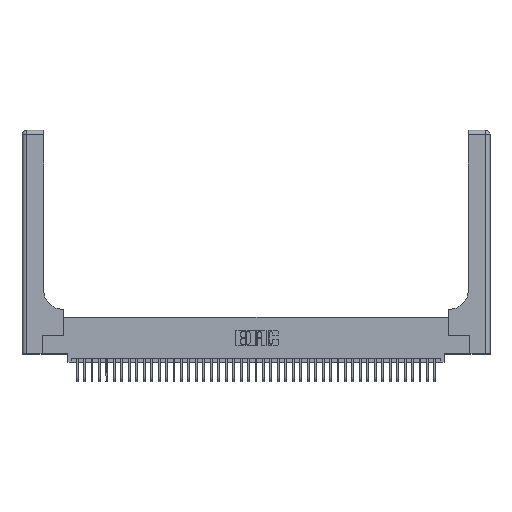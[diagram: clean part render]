
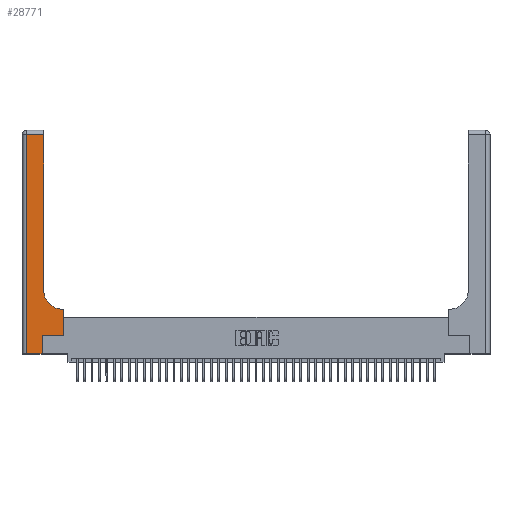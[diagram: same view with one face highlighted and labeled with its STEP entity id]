
A CAD part, top view. The second image highlights one B-rep face of the part: STEP entity #28771.
In plain terms, the highlighted planar face has unit normal (0, 0, 1).
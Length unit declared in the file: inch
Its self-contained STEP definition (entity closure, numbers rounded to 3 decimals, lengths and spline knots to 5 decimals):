
#1173 = VERTEX_POINT ( 'NONE', #17177 ) ;
#1456 = CARTESIAN_POINT ( 'NONE',  ( 0.269, 0., 0.37 ) ) ;
#2122 = CARTESIAN_POINT ( 'NONE',  ( 0., 0., 0.37 ) ) ;
#2748 = AXIS2_PLACEMENT_3D ( 'NONE', #17704, #24197, #4902 ) ;
#2827 = CARTESIAN_POINT ( 'NONE',  ( 0.2915, 2.94, 0.37 ) ) ;
#2954 = DIRECTION ( 'NONE',  ( 0., 0., -1. ) ) ;
#3810 = ORIENTED_EDGE ( 'NONE', *, *, #24860, .T. ) ;
#3880 = AXIS2_PLACEMENT_3D ( 'NONE', #22214, #2954, #25472 ) ;
#4697 = DIRECTION ( 'NONE',  ( 0., 1., 0. ) ) ;
#4902 = DIRECTION ( 'NONE',  ( -1., 0., 0. ) ) ;
#5010 = VECTOR ( 'NONE', #23954, 39.37008 ) ;
#5821 = CIRCLE ( 'NONE', #3880, 0.25 ) ;
#6373 = CARTESIAN_POINT ( 'NONE',  ( 0., 2.94, 0.37 ) ) ;
#6786 = VERTEX_POINT ( 'NONE', #27346 ) ;
#6791 = VERTEX_POINT ( 'NONE', #33698 ) ;
#7087 = LINE ( 'NONE', #31701, #14692 ) ;
#7318 = EDGE_CURVE ( 'NONE', #6791, #16129, #30686, .T. ) ;
#7446 = DIRECTION ( 'NONE',  ( -1., 0., 0. ) ) ;
#7979 = DIRECTION ( 'NONE',  ( 0., 1., 0. ) ) ;
#8116 = VECTOR ( 'NONE', #4697, 39.37008 ) ;
#11097 = CARTESIAN_POINT ( 'NONE',  ( 0.269, 0., 0.37 ) ) ;
#11249 = ORIENTED_EDGE ( 'NONE', *, *, #15814, .T. ) ;
#12452 = VERTEX_POINT ( 'NONE', #20300 ) ;
#13933 = CARTESIAN_POINT ( 'NONE',  ( 0.06, 0., 0.37 ) ) ;
#14692 = VECTOR ( 'NONE', #38036, 39.37008 ) ;
#14932 = CARTESIAN_POINT ( 'NONE',  ( 0.269, 0.25, 0.37 ) ) ;
#15590 = LINE ( 'NONE', #36550, #5010 ) ;
#15814 = EDGE_CURVE ( 'NONE', #19486, #25115, #34128, .T. ) ;
#15966 = ORIENTED_EDGE ( 'NONE', *, *, #19341, .T. ) ;
#16129 = VERTEX_POINT ( 'NONE', #39869 ) ;
#16688 = LINE ( 'NONE', #20718, #8116 ) ;
#16715 = ORIENTED_EDGE ( 'NONE', *, *, #25728, .T. ) ;
#17177 = CARTESIAN_POINT ( 'NONE',  ( 0.2915, 0.85, 0.37 ) ) ;
#17704 = CARTESIAN_POINT ( 'NONE',  ( 0., 3., 0.37 ) ) ;
#18617 = ORIENTED_EDGE ( 'NONE', *, *, #23401, .T. ) ;
#19324 = DIRECTION ( 'NONE',  ( -1., 0., 0. ) ) ;
#19341 = EDGE_CURVE ( 'NONE', #12452, #6786, #21742, .T. ) ;
#19433 = FACE_OUTER_BOUND ( 'NONE', #28794, .T. ) ;
#19486 = VERTEX_POINT ( 'NONE', #2827 ) ;
#19494 = EDGE_CURVE ( 'NONE', #6786, #6791, #7087, .T. ) ;
#19976 = CARTESIAN_POINT ( 'NONE',  ( 0.2915, 0.6, 0.37 ) ) ;
#20300 = CARTESIAN_POINT ( 'NONE',  ( 0.269, 0.25, 0.37 ) ) ;
#20718 = CARTESIAN_POINT ( 'NONE',  ( 0.2915, 3., 0.37 ) ) ;
#20791 = LINE ( 'NONE', #2122, #28329 ) ;
#21366 = DIRECTION ( 'NONE',  ( 1., 0., 0. ) ) ;
#21374 = DIRECTION ( 'NONE',  ( 1., 0., 0. ) ) ;
#21742 = LINE ( 'NONE', #14932, #29249 ) ;
#22132 = ORIENTED_EDGE ( 'NONE', *, *, #7318, .T. ) ;
#22187 = VECTOR ( 'NONE', #7446, 39.37008 ) ;
#22214 = CARTESIAN_POINT ( 'NONE',  ( 0.5415, 0.85, 0.37 ) ) ;
#23401 = EDGE_CURVE ( 'NONE', #16129, #1173, #5821, .T. ) ;
#23954 = DIRECTION ( 'NONE',  ( 0., -1., 0. ) ) ;
#24197 = DIRECTION ( 'NONE',  ( 0., 0., -1. ) ) ;
#24860 = EDGE_CURVE ( 'NONE', #29997, #12452, #25355, .T. ) ;
#25115 = VERTEX_POINT ( 'NONE', #41319 ) ;
#25355 = LINE ( 'NONE', #11097, #33752 ) ;
#25472 = DIRECTION ( 'NONE',  ( 1., 0., 0. ) ) ;
#25724 = VECTOR ( 'NONE', #19324, 39.37008 ) ;
#25728 = EDGE_CURVE ( 'NONE', #1173, #19486, #16688, .T. ) ;
#26934 = ORIENTED_EDGE ( 'NONE', *, *, #39657, .T. ) ;
#27346 = CARTESIAN_POINT ( 'NONE',  ( 0.5585, 0.25, 0.37 ) ) ;
#28329 = VECTOR ( 'NONE', #21366, 39.37008 ) ;
#28570 = ORIENTED_EDGE ( 'NONE', *, *, #19494, .T. ) ;
#28771 = ADVANCED_FACE ( 'NONE', ( #19433 ), #36786, .F. ) ;
#28794 = EDGE_LOOP ( 'NONE', ( #16715, #11249, #33198, #26934, #3810, #15966, #28570, #22132, #18617 ) ) ;
#29249 = VECTOR ( 'NONE', #21374, 39.37008 ) ;
#29997 = VERTEX_POINT ( 'NONE', #1456 ) ;
#30686 = LINE ( 'NONE', #19976, #22187 ) ;
#31701 = CARTESIAN_POINT ( 'NONE',  ( 0.5585, 0.25, 0.37 ) ) ;
#33198 = ORIENTED_EDGE ( 'NONE', *, *, #35290, .T. ) ;
#33698 = CARTESIAN_POINT ( 'NONE',  ( 0.5585, 0.6, 0.37 ) ) ;
#33752 = VECTOR ( 'NONE', #7979, 39.37008 ) ;
#34128 = LINE ( 'NONE', #6373, #25724 ) ;
#35290 = EDGE_CURVE ( 'NONE', #25115, #37760, #15590, .T. ) ;
#36550 = CARTESIAN_POINT ( 'NONE',  ( 0.06, 3., 0.37 ) ) ;
#36786 = PLANE ( 'NONE',  #2748 ) ;
#37760 = VERTEX_POINT ( 'NONE', #13933 ) ;
#38036 = DIRECTION ( 'NONE',  ( 0., 1., 0. ) ) ;
#39657 = EDGE_CURVE ( 'NONE', #37760, #29997, #20791, .T. ) ;
#39869 = CARTESIAN_POINT ( 'NONE',  ( 0.5415, 0.6, 0.37 ) ) ;
#41319 = CARTESIAN_POINT ( 'NONE',  ( 0.06, 2.94, 0.37 ) ) ;
